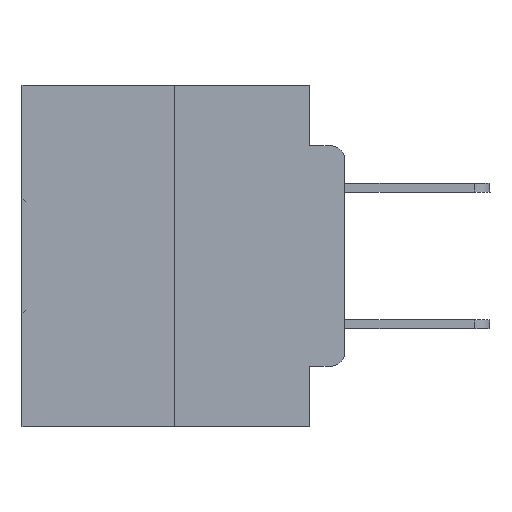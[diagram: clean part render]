
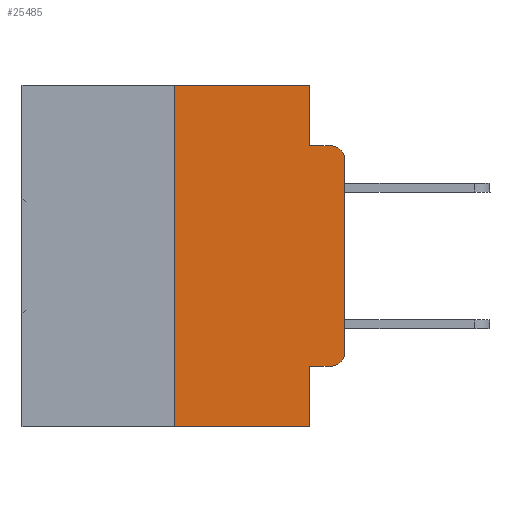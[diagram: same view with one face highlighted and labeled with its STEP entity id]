
A CAD part, left-side view. The second image highlights one B-rep face of the part: STEP entity #25485.
In plain terms, the highlighted planar face has unit normal (-1, 0, 0).
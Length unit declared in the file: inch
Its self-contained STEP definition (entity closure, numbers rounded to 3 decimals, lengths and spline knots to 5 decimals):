
#31 = CARTESIAN_POINT ( 'NONE',  ( 0., 0., -0.3915 ) ) ;
#342 = CARTESIAN_POINT ( 'NONE',  ( 0., 0.25, 0. ) ) ;
#817 = DIRECTION ( 'NONE',  ( 0., 0., -1. ) ) ;
#898 = LINE ( 'NONE', #6361, #11649 ) ;
#1308 = EDGE_CURVE ( 'NONE', #7303, #21294, #30234, .T. ) ;
#1635 = VERTEX_POINT ( 'NONE', #11534 ) ;
#1942 = EDGE_CURVE ( 'NONE', #16277, #1635, #6962, .T. ) ;
#2375 = AXIS2_PLACEMENT_3D ( 'NONE', #20665, #25620, #817 ) ;
#2973 = ORIENTED_EDGE ( 'NONE', *, *, #11280, .F. ) ;
#3085 = DIRECTION ( 'NONE',  ( -1., 0., 0. ) ) ;
#3111 = EDGE_CURVE ( 'NONE', #23331, #7303, #9599, .T. ) ;
#3426 = CARTESIAN_POINT ( 'NONE',  ( 0., 0.051, 0. ) ) ;
#3546 = DIRECTION ( 'NONE',  ( 0., -1., 0. ) ) ;
#3726 = CARTESIAN_POINT ( 'NONE',  ( 0., 0.051, -0.0885 ) ) ;
#5311 = VERTEX_POINT ( 'NONE', #3726 ) ;
#5570 = ORIENTED_EDGE ( 'NONE', *, *, #3111, .T. ) ;
#5799 = ORIENTED_EDGE ( 'NONE', *, *, #1308, .T. ) ;
#5816 = ORIENTED_EDGE ( 'NONE', *, *, #1942, .T. ) ;
#6361 = CARTESIAN_POINT ( 'NONE',  ( 0., 0.051, -0.4115 ) ) ;
#6962 = LINE ( 'NONE', #11893, #11981 ) ;
#7158 = ORIENTED_EDGE ( 'NONE', *, *, #24335, .F. ) ;
#7241 = EDGE_LOOP ( 'NONE', ( #5799, #29621, #11072, #2973, #7158, #30557, #5816, #11809, #19722, #5570 ) ) ;
#7303 = VERTEX_POINT ( 'NONE', #31 ) ;
#7403 = VERTEX_POINT ( 'NONE', #342 ) ;
#8121 = EDGE_CURVE ( 'NONE', #27699, #1635, #25441, .T. ) ;
#8576 = CARTESIAN_POINT ( 'NONE',  ( 0., 0.051, -0.4115 ) ) ;
#9599 = CIRCLE ( 'NONE', #2375, 0.02 ) ;
#10043 = CARTESIAN_POINT ( 'NONE',  ( 0., 0.051, 0. ) ) ;
#10270 = VECTOR ( 'NONE', #28024, 39.37008 ) ;
#11072 = ORIENTED_EDGE ( 'NONE', *, *, #31864, .F. ) ;
#11280 = EDGE_CURVE ( 'NONE', #21826, #5311, #21513, .T. ) ;
#11534 = CARTESIAN_POINT ( 'NONE',  ( 0., 0.051, -0.5 ) ) ;
#11649 = VECTOR ( 'NONE', #16287, 39.37008 ) ;
#11809 = ORIENTED_EDGE ( 'NONE', *, *, #8121, .F. ) ;
#11893 = CARTESIAN_POINT ( 'NONE',  ( 0., 0.473, -0.5 ) ) ;
#11981 = VECTOR ( 'NONE', #29208, 39.37008 ) ;
#12591 = EDGE_CURVE ( 'NONE', #21294, #15363, #29603, .T. ) ;
#12902 = DIRECTION ( 'NONE',  ( 0., 0., 1. ) ) ;
#13288 = CARTESIAN_POINT ( 'NONE',  ( 0., 0.02, -0.0885 ) ) ;
#13694 = LINE ( 'NONE', #29779, #27234 ) ;
#15354 = CARTESIAN_POINT ( 'NONE',  ( 0., 0.02, -0.1085 ) ) ;
#15363 = VERTEX_POINT ( 'NONE', #13288 ) ;
#16277 = VERTEX_POINT ( 'NONE', #24418 ) ;
#16287 = DIRECTION ( 'NONE',  ( 0., -1., 0. ) ) ;
#17794 = CARTESIAN_POINT ( 'NONE',  ( 0., 0.25, 0. ) ) ;
#17798 = CARTESIAN_POINT ( 'NONE',  ( 0., 0.051, 0. ) ) ;
#18480 = AXIS2_PLACEMENT_3D ( 'NONE', #15354, #3085, #22731 ) ;
#18974 = DIRECTION ( 'NONE',  ( 0., 0., 1. ) ) ;
#19385 = VECTOR ( 'NONE', #12902, 39.37008 ) ;
#19722 = ORIENTED_EDGE ( 'NONE', *, *, #31413, .T. ) ;
#19813 = FACE_OUTER_BOUND ( 'NONE', #7241, .T. ) ;
#20255 = DIRECTION ( 'NONE',  ( 0., -1., 0. ) ) ;
#20665 = CARTESIAN_POINT ( 'NONE',  ( 0., 0.02, -0.3915 ) ) ;
#21080 = AXIS2_PLACEMENT_3D ( 'NONE', #25375, #27741, #25155 ) ;
#21280 = CARTESIAN_POINT ( 'NONE',  ( 0., 0.02, -0.4115 ) ) ;
#21294 = VERTEX_POINT ( 'NONE', #24468 ) ;
#21513 = LINE ( 'NONE', #3426, #10270 ) ;
#21826 = VERTEX_POINT ( 'NONE', #17798 ) ;
#22485 = DIRECTION ( 'NONE',  ( 0., 0., -1. ) ) ;
#22731 = DIRECTION ( 'NONE',  ( 0., 0., -1. ) ) ;
#23331 = VERTEX_POINT ( 'NONE', #21280 ) ;
#24335 = EDGE_CURVE ( 'NONE', #7403, #21826, #13694, .T. ) ;
#24418 = CARTESIAN_POINT ( 'NONE',  ( 0., 0.25, -0.5 ) ) ;
#24468 = CARTESIAN_POINT ( 'NONE',  ( 0., 0., -0.1085 ) ) ;
#24952 = PLANE ( 'NONE',  #21080 ) ;
#25155 = DIRECTION ( 'NONE',  ( 0., 0., -1. ) ) ;
#25184 = LINE ( 'NONE', #17794, #19385 ) ;
#25375 = CARTESIAN_POINT ( 'NONE',  ( 0., 0.473, 0. ) ) ;
#25441 = LINE ( 'NONE', #10043, #28917 ) ;
#25485 = ADVANCED_FACE ( 'NONE', ( #19813 ), #24952, .F. ) ;
#25620 = DIRECTION ( 'NONE',  ( -1., 0., 0. ) ) ;
#27098 = VECTOR ( 'NONE', #3546, 39.37008 ) ;
#27234 = VECTOR ( 'NONE', #20255, 39.37008 ) ;
#27699 = VERTEX_POINT ( 'NONE', #8576 ) ;
#27741 = DIRECTION ( 'NONE',  ( 1., 0., 0. ) ) ;
#27869 = LINE ( 'NONE', #30967, #27098 ) ;
#28024 = DIRECTION ( 'NONE',  ( 0., 0., -1. ) ) ;
#28917 = VECTOR ( 'NONE', #22485, 39.37008 ) ;
#29208 = DIRECTION ( 'NONE',  ( 0., -1., 0. ) ) ;
#29603 = CIRCLE ( 'NONE', #18480, 0.02 ) ;
#29621 = ORIENTED_EDGE ( 'NONE', *, *, #12591, .T. ) ;
#29779 = CARTESIAN_POINT ( 'NONE',  ( 0., 0.473, 0. ) ) ;
#30234 = LINE ( 'NONE', #31747, #31799 ) ;
#30557 = ORIENTED_EDGE ( 'NONE', *, *, #31699, .F. ) ;
#30967 = CARTESIAN_POINT ( 'NONE',  ( 0., 0.051, -0.0885 ) ) ;
#31413 = EDGE_CURVE ( 'NONE', #27699, #23331, #898, .T. ) ;
#31699 = EDGE_CURVE ( 'NONE', #16277, #7403, #25184, .T. ) ;
#31747 = CARTESIAN_POINT ( 'NONE',  ( 0., 0., 0. ) ) ;
#31799 = VECTOR ( 'NONE', #18974, 39.37008 ) ;
#31864 = EDGE_CURVE ( 'NONE', #5311, #15363, #27869, .T. ) ;
